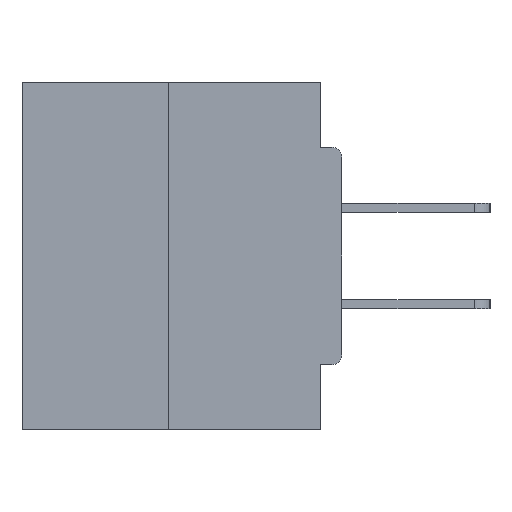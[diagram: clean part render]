
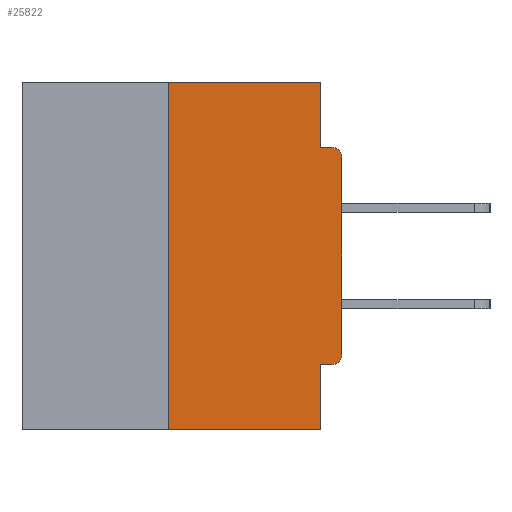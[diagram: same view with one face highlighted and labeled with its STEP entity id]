
A CAD part, left-side view. The second image highlights one B-rep face of the part: STEP entity #25822.
In plain terms, the highlighted planar face has unit normal (-1, 0, 0).
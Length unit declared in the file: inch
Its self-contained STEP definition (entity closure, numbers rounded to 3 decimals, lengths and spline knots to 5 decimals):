
#1131 = DIRECTION ( 'NONE',  ( -1., 0., 0. ) ) ;
#1582 = VERTEX_POINT ( 'NONE', #35634 ) ;
#1787 = LINE ( 'NONE', #31454, #23122 ) ;
#2652 = CIRCLE ( 'NONE', #30847, 0.015 ) ;
#3146 = EDGE_CURVE ( 'NONE', #9199, #32541, #32504, .T. ) ;
#3498 = DIRECTION ( 'NONE',  ( 0., 0., 1. ) ) ;
#3771 = CIRCLE ( 'NONE', #15298, 0.015 ) ;
#4134 = VECTOR ( 'NONE', #24204, 39.37008 ) ;
#5006 = CARTESIAN_POINT ( 'NONE',  ( 0., 0.46, 0. ) ) ;
#5128 = DIRECTION ( 'NONE',  ( 1., 0., 0. ) ) ;
#5143 = ORIENTED_EDGE ( 'NONE', *, *, #20253, .F. ) ;
#5284 = DIRECTION ( 'NONE',  ( 0., 0., 1. ) ) ;
#5383 = DIRECTION ( 'NONE',  ( 0., 0., -1. ) ) ;
#5422 = EDGE_CURVE ( 'NONE', #10428, #9125, #25334, .T. ) ;
#5475 = DIRECTION ( 'NONE',  ( 0., 0., -1. ) ) ;
#5826 = VERTEX_POINT ( 'NONE', #6067 ) ;
#6022 = ORIENTED_EDGE ( 'NONE', *, *, #31542, .T. ) ;
#6067 = CARTESIAN_POINT ( 'NONE',  ( 0., 0., -0.3915 ) ) ;
#6312 = ORIENTED_EDGE ( 'NONE', *, *, #26794, .F. ) ;
#6796 = CARTESIAN_POINT ( 'NONE',  ( 0., 0.46, 0. ) ) ;
#7119 = VERTEX_POINT ( 'NONE', #21739 ) ;
#7623 = FACE_OUTER_BOUND ( 'NONE', #26867, .T. ) ;
#8051 = LINE ( 'NONE', #8632, #23620 ) ;
#8064 = DIRECTION ( 'NONE',  ( -1., 0., 0. ) ) ;
#8632 = CARTESIAN_POINT ( 'NONE',  ( 0., 0., -0.0935 ) ) ;
#8654 = VERTEX_POINT ( 'NONE', #30671 ) ;
#8763 = ORIENTED_EDGE ( 'NONE', *, *, #30874, .F. ) ;
#8917 = LINE ( 'NONE', #23733, #24870 ) ;
#8994 = VERTEX_POINT ( 'NONE', #21857 ) ;
#9125 = VERTEX_POINT ( 'NONE', #11798 ) ;
#9199 = VERTEX_POINT ( 'NONE', #17509 ) ;
#10428 = VERTEX_POINT ( 'NONE', #15616 ) ;
#10833 = EDGE_CURVE ( 'NONE', #1582, #9199, #21092, .T. ) ;
#11316 = VECTOR ( 'NONE', #29487, 39.37008 ) ;
#11477 = DIRECTION ( 'NONE',  ( 0., -1., 0. ) ) ;
#11798 = CARTESIAN_POINT ( 'NONE',  ( 0., 0.031, -0.5 ) ) ;
#12016 = VECTOR ( 'NONE', #34562, 39.37008 ) ;
#12975 = VECTOR ( 'NONE', #5475, 39.37008 ) ;
#13636 = CARTESIAN_POINT ( 'NONE',  ( 0., 0.031, -0.5 ) ) ;
#13747 = CARTESIAN_POINT ( 'NONE',  ( 0., 0.015, -0.3915 ) ) ;
#15261 = CARTESIAN_POINT ( 'NONE',  ( 0., 0.015, -0.1085 ) ) ;
#15298 = AXIS2_PLACEMENT_3D ( 'NONE', #13747, #8064, #30727 ) ;
#15616 = CARTESIAN_POINT ( 'NONE',  ( 0., 0.25, -0.5 ) ) ;
#17020 = ORIENTED_EDGE ( 'NONE', *, *, #28137, .T. ) ;
#17509 = CARTESIAN_POINT ( 'NONE',  ( 0., 0.031, 0. ) ) ;
#18875 = ORIENTED_EDGE ( 'NONE', *, *, #3146, .F. ) ;
#19227 = ORIENTED_EDGE ( 'NONE', *, *, #35297, .T. ) ;
#19291 = CARTESIAN_POINT ( 'NONE',  ( 0., 0.25, 0. ) ) ;
#19374 = EDGE_CURVE ( 'NONE', #8994, #9125, #21424, .T. ) ;
#20253 = EDGE_CURVE ( 'NONE', #32541, #7119, #8051, .T. ) ;
#20861 = CARTESIAN_POINT ( 'NONE',  ( 0., 0.46, -0.5 ) ) ;
#20977 = DIRECTION ( 'NONE',  ( 0., 0., -1. ) ) ;
#21092 = LINE ( 'NONE', #6796, #11316 ) ;
#21424 = LINE ( 'NONE', #13636, #12975 ) ;
#21659 = ORIENTED_EDGE ( 'NONE', *, *, #5422, .T. ) ;
#21739 = CARTESIAN_POINT ( 'NONE',  ( 0., 0.015, -0.0935 ) ) ;
#21857 = CARTESIAN_POINT ( 'NONE',  ( 0., 0.031, -0.4065 ) ) ;
#22083 = ORIENTED_EDGE ( 'NONE', *, *, #19374, .F. ) ;
#23122 = VECTOR ( 'NONE', #25788, 39.37008 ) ;
#23620 = VECTOR ( 'NONE', #11477, 39.37008 ) ;
#23733 = CARTESIAN_POINT ( 'NONE',  ( 0., 0., 0. ) ) ;
#24204 = DIRECTION ( 'NONE',  ( 0., 0., -1. ) ) ;
#24870 = VECTOR ( 'NONE', #3498, 39.37008 ) ;
#24876 = ORIENTED_EDGE ( 'NONE', *, *, #10833, .F. ) ;
#25334 = LINE ( 'NONE', #20861, #12016 ) ;
#25788 = DIRECTION ( 'NONE',  ( 0., 1., 0. ) ) ;
#25822 = ADVANCED_FACE ( 'NONE', ( #7623 ), #36111, .F. ) ;
#25843 = AXIS2_PLACEMENT_3D ( 'NONE', #5006, #5128, #5383 ) ;
#26509 = LINE ( 'NONE', #19291, #36180 ) ;
#26794 = EDGE_CURVE ( 'NONE', #8654, #8994, #1787, .T. ) ;
#26867 = EDGE_LOOP ( 'NONE', ( #24876, #8763, #21659, #22083, #6312, #6022, #19227, #17020, #5143, #18875 ) ) ;
#28137 = EDGE_CURVE ( 'NONE', #31293, #7119, #2652, .T. ) ;
#29304 = CARTESIAN_POINT ( 'NONE',  ( 0., 0., -0.1085 ) ) ;
#29487 = DIRECTION ( 'NONE',  ( 0., -1., 0. ) ) ;
#30597 = CARTESIAN_POINT ( 'NONE',  ( 0., 0.031, -0.0935 ) ) ;
#30671 = CARTESIAN_POINT ( 'NONE',  ( 0., 0.015, -0.4065 ) ) ;
#30727 = DIRECTION ( 'NONE',  ( 0., 0., -1. ) ) ;
#30847 = AXIS2_PLACEMENT_3D ( 'NONE', #15261, #1131, #20977 ) ;
#30874 = EDGE_CURVE ( 'NONE', #10428, #1582, #26509, .T. ) ;
#31293 = VERTEX_POINT ( 'NONE', #29304 ) ;
#31454 = CARTESIAN_POINT ( 'NONE',  ( 0., 0., -0.4065 ) ) ;
#31542 = EDGE_CURVE ( 'NONE', #8654, #5826, #3771, .T. ) ;
#32504 = LINE ( 'NONE', #32823, #4134 ) ;
#32541 = VERTEX_POINT ( 'NONE', #30597 ) ;
#32823 = CARTESIAN_POINT ( 'NONE',  ( 0., 0.031, 0. ) ) ;
#34562 = DIRECTION ( 'NONE',  ( 0., -1., 0. ) ) ;
#35297 = EDGE_CURVE ( 'NONE', #5826, #31293, #8917, .T. ) ;
#35634 = CARTESIAN_POINT ( 'NONE',  ( 0., 0.25, 0. ) ) ;
#36111 = PLANE ( 'NONE',  #25843 ) ;
#36180 = VECTOR ( 'NONE', #5284, 39.37008 ) ;
